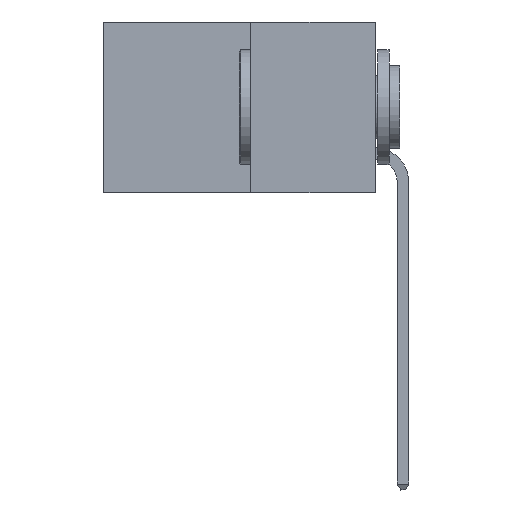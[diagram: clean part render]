
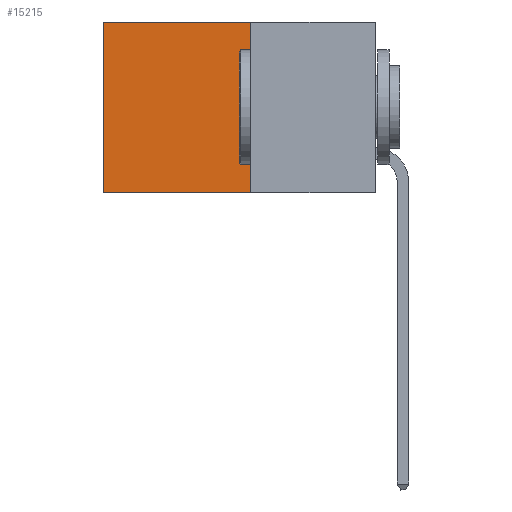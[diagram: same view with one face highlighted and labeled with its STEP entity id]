
A CAD part, left-side view. The second image highlights one B-rep face of the part: STEP entity #15215.
In plain terms, the highlighted planar face has unit normal (-1, 0, 0).
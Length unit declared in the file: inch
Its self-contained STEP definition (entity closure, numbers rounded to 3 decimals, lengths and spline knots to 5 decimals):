
#354 = AXIS2_PLACEMENT_3D ( 'NONE', #27376, #14165, #802 ) ;
#546 = VERTEX_POINT ( 'NONE', #6872 ) ;
#802 = DIRECTION ( 'NONE',  ( 0., 0., -1. ) ) ;
#810 = LINE ( 'NONE', #26022, #23729 ) ;
#4177 = ORIENTED_EDGE ( 'NONE', *, *, #13337, .T. ) ;
#4279 = FACE_OUTER_BOUND ( 'NONE', #16325, .T. ) ;
#5828 = DIRECTION ( 'NONE',  ( 0., 0., -1. ) ) ;
#6872 = CARTESIAN_POINT ( 'NONE',  ( 0.277, 0.59, -0.37 ) ) ;
#7115 = LINE ( 'NONE', #20610, #28556 ) ;
#7128 = EDGE_CURVE ( 'NONE', #12449, #9691, #7115, .T. ) ;
#7946 = EDGE_CURVE ( 'NONE', #9691, #546, #26430, .T. ) ;
#9691 = VERTEX_POINT ( 'NONE', #26445 ) ;
#9811 = CARTESIAN_POINT ( 'NONE',  ( 0.277, 0.59, -0.37 ) ) ;
#11846 = CARTESIAN_POINT ( 'NONE',  ( 0.277, 0.27, -0.37 ) ) ;
#12027 = DIRECTION ( 'NONE',  ( 0., 0., -1. ) ) ;
#12449 = VERTEX_POINT ( 'NONE', #13424 ) ;
#13337 = EDGE_CURVE ( 'NONE', #18041, #546, #15866, .T. ) ;
#13424 = CARTESIAN_POINT ( 'NONE',  ( 0.277, 0.27, 0. ) ) ;
#14165 = DIRECTION ( 'NONE',  ( 1., 0., 0. ) ) ;
#15215 = ADVANCED_FACE ( 'NONE', ( #4279 ), #25160, .F. ) ;
#15866 = LINE ( 'NONE', #9811, #26236 ) ;
#16325 = EDGE_LOOP ( 'NONE', ( #4177, #24452, #20699, #22186 ) ) ;
#18041 = VERTEX_POINT ( 'NONE', #18716 ) ;
#18716 = CARTESIAN_POINT ( 'NONE',  ( 0.277, 0.59, 0. ) ) ;
#20511 = VECTOR ( 'NONE', #27339, 39.37008 ) ;
#20610 = CARTESIAN_POINT ( 'NONE',  ( 0.277, 0.27, -0.37 ) ) ;
#20699 = ORIENTED_EDGE ( 'NONE', *, *, #7128, .F. ) ;
#21660 = DIRECTION ( 'NONE',  ( 0., 1., 0. ) ) ;
#22186 = ORIENTED_EDGE ( 'NONE', *, *, #24799, .T. ) ;
#23729 = VECTOR ( 'NONE', #21660, 39.37008 ) ;
#24452 = ORIENTED_EDGE ( 'NONE', *, *, #7946, .F. ) ;
#24799 = EDGE_CURVE ( 'NONE', #12449, #18041, #810, .T. ) ;
#25160 = PLANE ( 'NONE',  #354 ) ;
#26022 = CARTESIAN_POINT ( 'NONE',  ( 0.277, 0.27, 0. ) ) ;
#26236 = VECTOR ( 'NONE', #12027, 39.37008 ) ;
#26430 = LINE ( 'NONE', #11846, #20511 ) ;
#26445 = CARTESIAN_POINT ( 'NONE',  ( 0.277, 0.27, -0.37 ) ) ;
#27339 = DIRECTION ( 'NONE',  ( 0., 1., 0. ) ) ;
#27376 = CARTESIAN_POINT ( 'NONE',  ( 0.277, 0.27, -0.37 ) ) ;
#28556 = VECTOR ( 'NONE', #5828, 39.37008 ) ;
